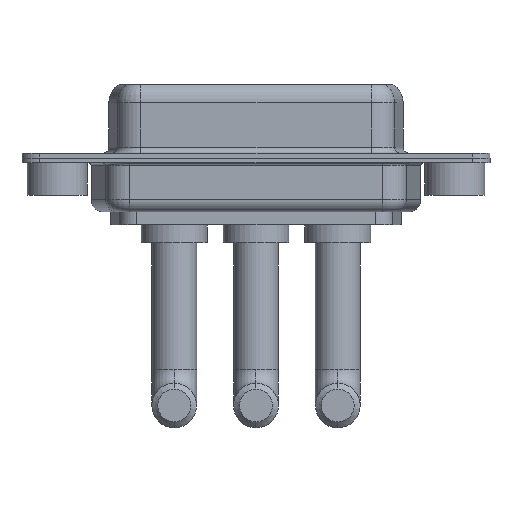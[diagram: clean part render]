
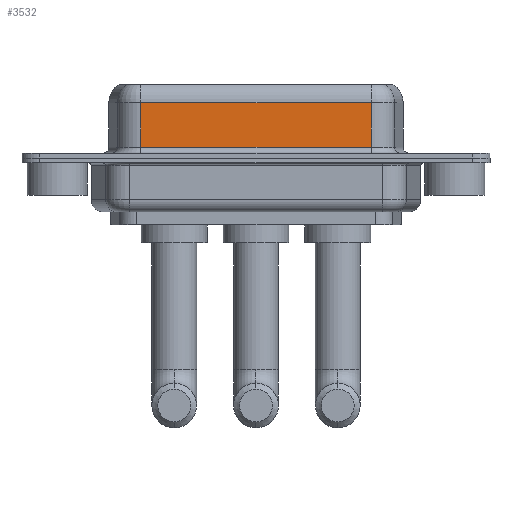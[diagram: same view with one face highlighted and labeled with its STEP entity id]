
A CAD part, front view. The second image highlights one B-rep face of the part: STEP entity #3532.
In plain terms, the highlighted planar face has unit normal (0, -1, 0).
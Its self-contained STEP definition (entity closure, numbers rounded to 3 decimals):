
#55 = ORIENTED_EDGE ( 'NONE', *, *, #6723, .F. ) ;
#363 = AXIS2_PLACEMENT_3D ( 'NONE', #11877, #11116, #6207 ) ;
#1004 = ORIENTED_EDGE ( 'NONE', *, *, #8936, .T. ) ;
#1238 = LINE ( 'NONE', #5321, #3665 ) ;
#1324 = EDGE_CURVE ( 'NONE', #11680, #3669, #1238, .T. ) ;
#1354 = EDGE_CURVE ( 'NONE', #3669, #8976, #5386, .T. ) ;
#1797 = CARTESIAN_POINT ( 'NONE',  ( 7.013, -3.95, 0.9 ) ) ;
#2012 = VECTOR ( 'NONE', #6458, 1000. ) ;
#2496 = DIRECTION ( 'NONE',  ( 0., 0., -1. ) ) ;
#2510 = LINE ( 'NONE', #3432, #2012 ) ;
#3432 = CARTESIAN_POINT ( 'NONE',  ( 26.287, -3.95, 4.65 ) ) ;
#3532 = ADVANCED_FACE ( 'NONE', ( #7227 ), #9204, .F. ) ;
#3665 = VECTOR ( 'NONE', #2496, 1000. ) ;
#3669 = VERTEX_POINT ( 'NONE', #1797 ) ;
#5055 = VECTOR ( 'NONE', #6384, 1000. ) ;
#5220 = CARTESIAN_POINT ( 'NONE',  ( 26.287, -3.95, 0.9 ) ) ;
#5321 = CARTESIAN_POINT ( 'NONE',  ( 7.013, -3.95, 6.4 ) ) ;
#5386 = LINE ( 'NONE', #7336, #5055 ) ;
#6207 = DIRECTION ( 'NONE',  ( 0., 0., 1. ) ) ;
#6365 = DIRECTION ( 'NONE',  ( 0., 0., -1. ) ) ;
#6384 = DIRECTION ( 'NONE',  ( 1., 0., 0. ) ) ;
#6458 = DIRECTION ( 'NONE',  ( -1., 0., 0. ) ) ;
#6652 = EDGE_LOOP ( 'NONE', ( #55, #1004, #9757, #9070 ) ) ;
#6723 = EDGE_CURVE ( 'NONE', #11995, #8976, #9295, .T. ) ;
#6782 = VECTOR ( 'NONE', #6365, 1000. ) ;
#7227 = FACE_OUTER_BOUND ( 'NONE', #6652, .T. ) ;
#7336 = CARTESIAN_POINT ( 'NONE',  ( 26.287, -3.95, 0.9 ) ) ;
#8362 = CARTESIAN_POINT ( 'NONE',  ( 26.287, -3.95, 6.4 ) ) ;
#8936 = EDGE_CURVE ( 'NONE', #11995, #11680, #2510, .T. ) ;
#8976 = VERTEX_POINT ( 'NONE', #5220 ) ;
#9070 = ORIENTED_EDGE ( 'NONE', *, *, #1354, .T. ) ;
#9204 = PLANE ( 'NONE',  #363 ) ;
#9295 = LINE ( 'NONE', #8362, #6782 ) ;
#9757 = ORIENTED_EDGE ( 'NONE', *, *, #1324, .T. ) ;
#9972 = CARTESIAN_POINT ( 'NONE',  ( 7.013, -3.95, 4.65 ) ) ;
#10474 = CARTESIAN_POINT ( 'NONE',  ( 26.287, -3.95, 4.65 ) ) ;
#11116 = DIRECTION ( 'NONE',  ( 0., 1., 0. ) ) ;
#11680 = VERTEX_POINT ( 'NONE', #9972 ) ;
#11877 = CARTESIAN_POINT ( 'NONE',  ( 26.287, -3.95, 6.4 ) ) ;
#11995 = VERTEX_POINT ( 'NONE', #10474 ) ;
